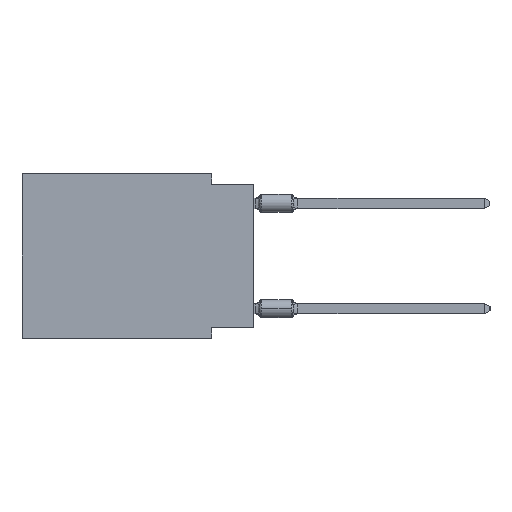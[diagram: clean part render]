
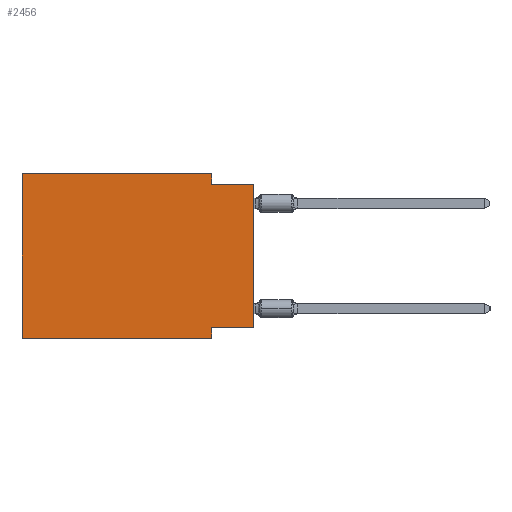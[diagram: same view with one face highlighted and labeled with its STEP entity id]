
A CAD part, left-side view. The second image highlights one B-rep face of the part: STEP entity #2456.
In plain terms, the highlighted planar face has unit normal (-1, 0, 0).
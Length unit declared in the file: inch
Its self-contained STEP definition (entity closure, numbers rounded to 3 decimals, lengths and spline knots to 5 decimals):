
#77 = AXIS2_PLACEMENT_3D ( 'NONE', #9148, #24965, #12145 ) ;
#1136 = VECTOR ( 'NONE', #16348, 39.37008 ) ;
#2456 = ADVANCED_FACE ( 'NONE', ( #24161 ), #39591, .F. ) ;
#2826 = DIRECTION ( 'NONE',  ( 0., -1., 0. ) ) ;
#3504 = CARTESIAN_POINT ( 'NONE',  ( 0., 0.55, -0.39 ) ) ;
#4235 = VECTOR ( 'NONE', #30399, 39.37008 ) ;
#4291 = CARTESIAN_POINT ( 'NONE',  ( 0., 0., -0.025 ) ) ;
#4490 = EDGE_CURVE ( 'NONE', #29130, #13165, #24283, .T. ) ;
#5328 = DIRECTION ( 'NONE',  ( 0., 1., 0. ) ) ;
#5436 = LINE ( 'NONE', #8452, #34207 ) ;
#5554 = CARTESIAN_POINT ( 'NONE',  ( 0., 0.1, 0. ) ) ;
#6262 = ORIENTED_EDGE ( 'NONE', *, *, #38836, .F. ) ;
#6773 = VERTEX_POINT ( 'NONE', #23961 ) ;
#7121 = EDGE_CURVE ( 'NONE', #22416, #30115, #5436, .T. ) ;
#7259 = ORIENTED_EDGE ( 'NONE', *, *, #7121, .F. ) ;
#7356 = ORIENTED_EDGE ( 'NONE', *, *, #28388, .F. ) ;
#7536 = DIRECTION ( 'NONE',  ( 0., 0., 1. ) ) ;
#8301 = ORIENTED_EDGE ( 'NONE', *, *, #4490, .T. ) ;
#8452 = CARTESIAN_POINT ( 'NONE',  ( 0., 0.55, 0. ) ) ;
#8832 = ORIENTED_EDGE ( 'NONE', *, *, #22707, .T. ) ;
#8940 = EDGE_LOOP ( 'NONE', ( #8301, #20126, #32353, #7259, #25524, #8832, #7356, #6262 ) ) ;
#9148 = CARTESIAN_POINT ( 'NONE',  ( 0., 0.55, 0. ) ) ;
#9337 = LINE ( 'NONE', #3504, #4235 ) ;
#12145 = DIRECTION ( 'NONE',  ( 0., 0., -1. ) ) ;
#13165 = VERTEX_POINT ( 'NONE', #15798 ) ;
#14105 = EDGE_CURVE ( 'NONE', #30115, #34084, #21596, .T. ) ;
#14565 = CARTESIAN_POINT ( 'NONE',  ( 0., 0.1, 0. ) ) ;
#15654 = EDGE_CURVE ( 'NONE', #6773, #22416, #35414, .T. ) ;
#15798 = CARTESIAN_POINT ( 'NONE',  ( 0., 0., -0.025 ) ) ;
#16348 = DIRECTION ( 'NONE',  ( 0., -1., 0. ) ) ;
#16608 = CARTESIAN_POINT ( 'NONE',  ( 0., 0.55, 0. ) ) ;
#17900 = VECTOR ( 'NONE', #26778, 39.37008 ) ;
#18749 = VERTEX_POINT ( 'NONE', #39599 ) ;
#19284 = VECTOR ( 'NONE', #5328, 39.37008 ) ;
#20126 = ORIENTED_EDGE ( 'NONE', *, *, #34515, .F. ) ;
#20392 = LINE ( 'NONE', #29621, #19284 ) ;
#21596 = LINE ( 'NONE', #5554, #34727 ) ;
#22416 = VERTEX_POINT ( 'NONE', #16608 ) ;
#22707 = EDGE_CURVE ( 'NONE', #6773, #33676, #9337, .T. ) ;
#23752 = LINE ( 'NONE', #35797, #17900 ) ;
#23961 = CARTESIAN_POINT ( 'NONE',  ( 0., 0.55, -0.39 ) ) ;
#24161 = FACE_OUTER_BOUND ( 'NONE', #8940, .T. ) ;
#24283 = LINE ( 'NONE', #31482, #38165 ) ;
#24965 = DIRECTION ( 'NONE',  ( 1., 0., 0. ) ) ;
#25138 = VECTOR ( 'NONE', #7536, 39.37008 ) ;
#25524 = ORIENTED_EDGE ( 'NONE', *, *, #15654, .F. ) ;
#26778 = DIRECTION ( 'NONE',  ( 0., 0., -1. ) ) ;
#28065 = DIRECTION ( 'NONE',  ( 0., 0., 1. ) ) ;
#28388 = EDGE_CURVE ( 'NONE', #18749, #33676, #23752, .T. ) ;
#29130 = VERTEX_POINT ( 'NONE', #32316 ) ;
#29621 = CARTESIAN_POINT ( 'NONE',  ( 0., 0., -0.365 ) ) ;
#30115 = VERTEX_POINT ( 'NONE', #14565 ) ;
#30247 = DIRECTION ( 'NONE',  ( 0., 0., -1. ) ) ;
#30399 = DIRECTION ( 'NONE',  ( 0., -1., 0. ) ) ;
#31482 = CARTESIAN_POINT ( 'NONE',  ( 0., 0., 0. ) ) ;
#31744 = CARTESIAN_POINT ( 'NONE',  ( 0., 0.1, -0.39 ) ) ;
#31989 = LINE ( 'NONE', #4291, #1136 ) ;
#32040 = CARTESIAN_POINT ( 'NONE',  ( 0., 0.1, -0.025 ) ) ;
#32227 = CARTESIAN_POINT ( 'NONE',  ( 0., 0.55, 0. ) ) ;
#32316 = CARTESIAN_POINT ( 'NONE',  ( 0., 0., -0.365 ) ) ;
#32353 = ORIENTED_EDGE ( 'NONE', *, *, #14105, .F. ) ;
#33676 = VERTEX_POINT ( 'NONE', #31744 ) ;
#34084 = VERTEX_POINT ( 'NONE', #32040 ) ;
#34207 = VECTOR ( 'NONE', #2826, 39.37008 ) ;
#34515 = EDGE_CURVE ( 'NONE', #34084, #13165, #31989, .T. ) ;
#34727 = VECTOR ( 'NONE', #30247, 39.37008 ) ;
#35414 = LINE ( 'NONE', #32227, #25138 ) ;
#35797 = CARTESIAN_POINT ( 'NONE',  ( 0., 0.1, -0.39 ) ) ;
#38165 = VECTOR ( 'NONE', #28065, 39.37008 ) ;
#38836 = EDGE_CURVE ( 'NONE', #29130, #18749, #20392, .T. ) ;
#39591 = PLANE ( 'NONE',  #77 ) ;
#39599 = CARTESIAN_POINT ( 'NONE',  ( 0., 0.1, -0.365 ) ) ;
